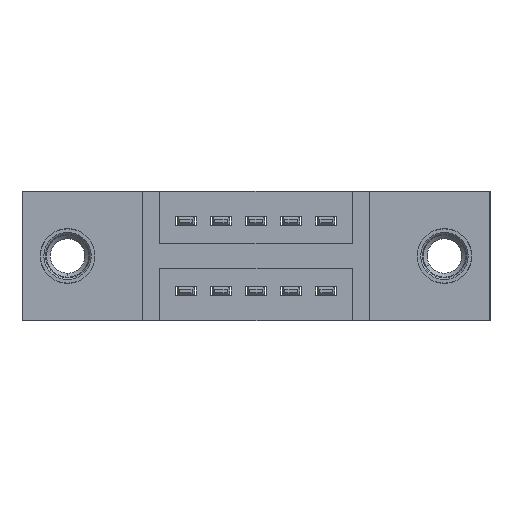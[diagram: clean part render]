
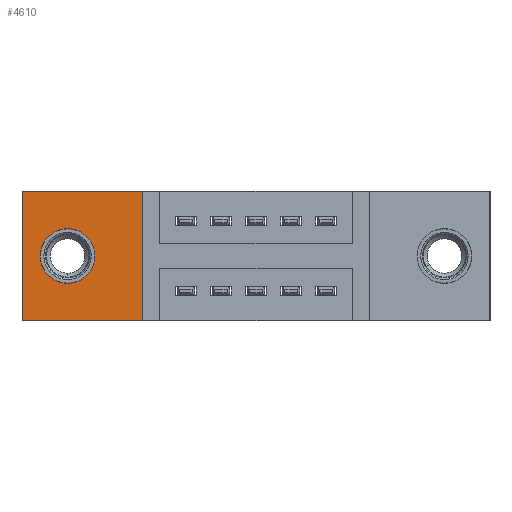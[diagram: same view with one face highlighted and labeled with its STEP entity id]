
A CAD part, front view. The second image highlights one B-rep face of the part: STEP entity #4610.
In plain terms, the highlighted planar face has unit normal (0, -1, 0).
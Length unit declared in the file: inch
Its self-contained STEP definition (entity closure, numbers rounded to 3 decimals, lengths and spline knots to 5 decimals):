
#84 = CARTESIAN_POINT ( 'NONE',  ( 0., 0.11, 0. ) ) ;
#91 = CARTESIAN_POINT ( 'NONE',  ( 0., 0.11, 0. ) ) ;
#212 = CARTESIAN_POINT ( 'NONE',  ( 0., 0.11, -0.37 ) ) ;
#238 = VECTOR ( 'NONE', #2407, 39.37008 ) ;
#425 = CARTESIAN_POINT ( 'NONE',  ( 0., 0.11, -0.37 ) ) ;
#591 = FACE_OUTER_BOUND ( 'NONE', #1792, .T. ) ;
#599 = ORIENTED_EDGE ( 'NONE', *, *, #7703, .T. ) ;
#691 = EDGE_CURVE ( 'NONE', #1104, #9858, #1488, .T. ) ;
#754 = AXIS2_PLACEMENT_3D ( 'NONE', #7005, #4595, #5380 ) ;
#854 = CARTESIAN_POINT ( 'NONE',  ( 0.13, 0.11, -0.263 ) ) ;
#1104 = VERTEX_POINT ( 'NONE', #1317 ) ;
#1317 = CARTESIAN_POINT ( 'NONE',  ( 0.13, 0.11, -0.107 ) ) ;
#1398 = AXIS2_PLACEMENT_3D ( 'NONE', #6675, #1998, #8434 ) ;
#1488 = CIRCLE ( 'NONE', #1398, 0.078 ) ;
#1644 = EDGE_CURVE ( 'NONE', #7309, #9295, #4765, .T. ) ;
#1667 = VERTEX_POINT ( 'NONE', #5422 ) ;
#1792 = EDGE_LOOP ( 'NONE', ( #7269, #599, #4717, #2926 ) ) ;
#1808 = CARTESIAN_POINT ( 'NONE',  ( 0.3425, 0.11, -0.37 ) ) ;
#1998 = DIRECTION ( 'NONE',  ( 0., -1., 0. ) ) ;
#2407 = DIRECTION ( 'NONE',  ( 0., 0., 1. ) ) ;
#2615 = ORIENTED_EDGE ( 'NONE', *, *, #691, .F. ) ;
#2739 = EDGE_CURVE ( 'NONE', #9858, #1104, #9938, .T. ) ;
#2926 = ORIENTED_EDGE ( 'NONE', *, *, #8177, .T. ) ;
#3017 = DIRECTION ( 'NONE',  ( 0., 0., -1. ) ) ;
#3430 = LINE ( 'NONE', #84, #5270 ) ;
#3556 = VERTEX_POINT ( 'NONE', #425 ) ;
#3879 = DIRECTION ( 'NONE',  ( 0., 0., -1. ) ) ;
#3987 = EDGE_CURVE ( 'NONE', #1667, #3556, #9495, .T. ) ;
#4086 = AXIS2_PLACEMENT_3D ( 'NONE', #9260, #5342, #3017 ) ;
#4595 = DIRECTION ( 'NONE',  ( 0., -1., 0. ) ) ;
#4610 = ADVANCED_FACE ( 'NONE', ( #5706, #591 ), #7713, .T. ) ;
#4717 = ORIENTED_EDGE ( 'NONE', *, *, #1644, .T. ) ;
#4754 = DIRECTION ( 'NONE',  ( 1., 0., 0. ) ) ;
#4765 = LINE ( 'NONE', #7796, #238 ) ;
#5270 = VECTOR ( 'NONE', #7010, 39.37008 ) ;
#5342 = DIRECTION ( 'NONE',  ( 0., -1., 0. ) ) ;
#5380 = DIRECTION ( 'NONE',  ( 0., 0., -1. ) ) ;
#5422 = CARTESIAN_POINT ( 'NONE',  ( 0., 0.11, 0. ) ) ;
#5706 = FACE_BOUND ( 'NONE', #6141, .T. ) ;
#6141 = EDGE_LOOP ( 'NONE', ( #2615, #8206 ) ) ;
#6286 = CARTESIAN_POINT ( 'NONE',  ( 0.3425, 0.11, 0. ) ) ;
#6675 = CARTESIAN_POINT ( 'NONE',  ( 0.13, 0.11, -0.185 ) ) ;
#7005 = CARTESIAN_POINT ( 'NONE',  ( 0.13, 0.11, -0.185 ) ) ;
#7010 = DIRECTION ( 'NONE',  ( -1., 0., 0. ) ) ;
#7211 = VECTOR ( 'NONE', #3879, 39.37008 ) ;
#7269 = ORIENTED_EDGE ( 'NONE', *, *, #3987, .T. ) ;
#7309 = VERTEX_POINT ( 'NONE', #1808 ) ;
#7591 = LINE ( 'NONE', #212, #9873 ) ;
#7703 = EDGE_CURVE ( 'NONE', #3556, #7309, #7591, .T. ) ;
#7713 = PLANE ( 'NONE',  #4086 ) ;
#7796 = CARTESIAN_POINT ( 'NONE',  ( 0.3425, 0.11, 0. ) ) ;
#8177 = EDGE_CURVE ( 'NONE', #9295, #1667, #3430, .T. ) ;
#8206 = ORIENTED_EDGE ( 'NONE', *, *, #2739, .F. ) ;
#8434 = DIRECTION ( 'NONE',  ( 0., 0., -1. ) ) ;
#9260 = CARTESIAN_POINT ( 'NONE',  ( 0., 0.11, -0.37 ) ) ;
#9295 = VERTEX_POINT ( 'NONE', #6286 ) ;
#9495 = LINE ( 'NONE', #91, #7211 ) ;
#9858 = VERTEX_POINT ( 'NONE', #854 ) ;
#9873 = VECTOR ( 'NONE', #4754, 39.37008 ) ;
#9938 = CIRCLE ( 'NONE', #754, 0.078 ) ;
